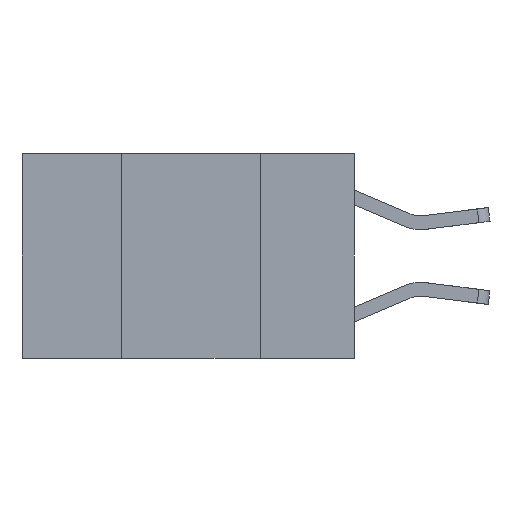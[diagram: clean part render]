
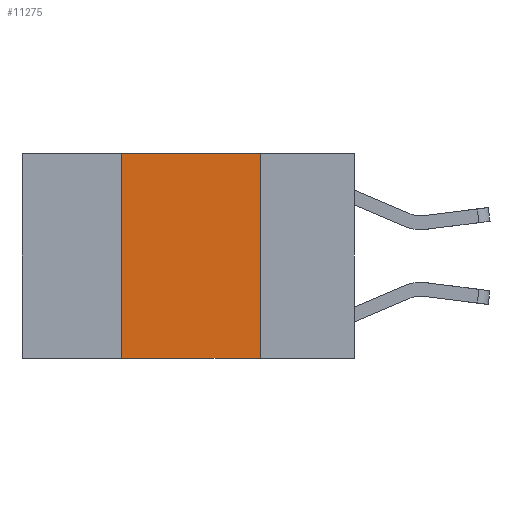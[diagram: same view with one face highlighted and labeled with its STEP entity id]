
A CAD part, left-side view. The second image highlights one B-rep face of the part: STEP entity #11275.
In plain terms, the highlighted planar face has unit normal (-1, 0, 0).
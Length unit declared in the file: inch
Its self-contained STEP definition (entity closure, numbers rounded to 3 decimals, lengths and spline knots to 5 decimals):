
#6 = VECTOR ( 'NONE', #7608, 39.37008 ) ;
#78 = VECTOR ( 'NONE', #3288, 39.37008 ) ;
#286 = LINE ( 'NONE', #1372, #9242 ) ;
#691 = DIRECTION ( 'NONE',  ( 0., -1., 0. ) ) ;
#1012 = CARTESIAN_POINT ( 'NONE',  ( 0., 0.6, 0. ) ) ;
#1372 = CARTESIAN_POINT ( 'NONE',  ( 0., 0.6, -0.37 ) ) ;
#1415 = CARTESIAN_POINT ( 'NONE',  ( 0., 0.17, 0. ) ) ;
#1587 = ORIENTED_EDGE ( 'NONE', *, *, #11061, .F. ) ;
#1922 = DIRECTION ( 'NONE',  ( 0., 0., -1. ) ) ;
#1999 = CARTESIAN_POINT ( 'NONE',  ( 0., 0.17, 0. ) ) ;
#2067 = CARTESIAN_POINT ( 'NONE',  ( 0., 0.42, 0. ) ) ;
#2187 = VECTOR ( 'NONE', #6749, 39.37008 ) ;
#2424 = LINE ( 'NONE', #2067, #6 ) ;
#2494 = LINE ( 'NONE', #5832, #2187 ) ;
#2764 = VERTEX_POINT ( 'NONE', #10281 ) ;
#3026 = EDGE_LOOP ( 'NONE', ( #1587, #6618, #10838, #9008 ) ) ;
#3265 = EDGE_CURVE ( 'NONE', #8100, #2764, #286, .T. ) ;
#3288 = DIRECTION ( 'NONE',  ( 0., 0., -1. ) ) ;
#3841 = CARTESIAN_POINT ( 'NONE',  ( 0., 0.42, 0. ) ) ;
#5063 = LINE ( 'NONE', #1415, #78 ) ;
#5113 = AXIS2_PLACEMENT_3D ( 'NONE', #1012, #7478, #1922 ) ;
#5285 = EDGE_CURVE ( 'NONE', #10843, #9197, #2494, .T. ) ;
#5832 = CARTESIAN_POINT ( 'NONE',  ( 0., 0.6, 0. ) ) ;
#6439 = EDGE_CURVE ( 'NONE', #8100, #10843, #2424, .T. ) ;
#6618 = ORIENTED_EDGE ( 'NONE', *, *, #5285, .F. ) ;
#6647 = PLANE ( 'NONE',  #5113 ) ;
#6749 = DIRECTION ( 'NONE',  ( 0., -1., 0. ) ) ;
#6787 = FACE_OUTER_BOUND ( 'NONE', #3026, .T. ) ;
#7327 = CARTESIAN_POINT ( 'NONE',  ( 0., 0.42, -0.37 ) ) ;
#7478 = DIRECTION ( 'NONE',  ( 1., 0., 0. ) ) ;
#7608 = DIRECTION ( 'NONE',  ( 0., 0., 1. ) ) ;
#8100 = VERTEX_POINT ( 'NONE', #7327 ) ;
#9008 = ORIENTED_EDGE ( 'NONE', *, *, #3265, .T. ) ;
#9197 = VERTEX_POINT ( 'NONE', #1999 ) ;
#9242 = VECTOR ( 'NONE', #691, 39.37008 ) ;
#10281 = CARTESIAN_POINT ( 'NONE',  ( 0., 0.17, -0.37 ) ) ;
#10838 = ORIENTED_EDGE ( 'NONE', *, *, #6439, .F. ) ;
#10843 = VERTEX_POINT ( 'NONE', #3841 ) ;
#11061 = EDGE_CURVE ( 'NONE', #9197, #2764, #5063, .T. ) ;
#11275 = ADVANCED_FACE ( 'NONE', ( #6787 ), #6647, .F. ) ;
